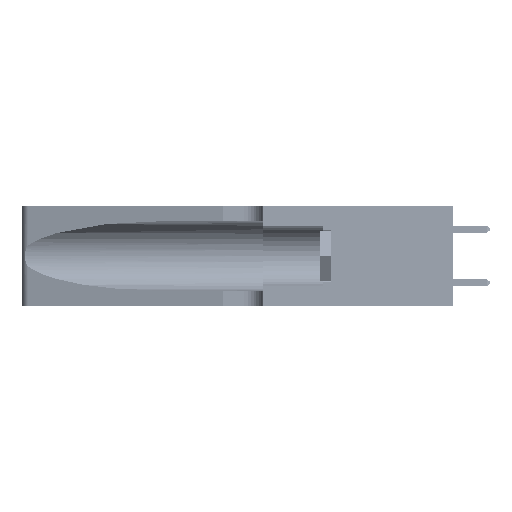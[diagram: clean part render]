
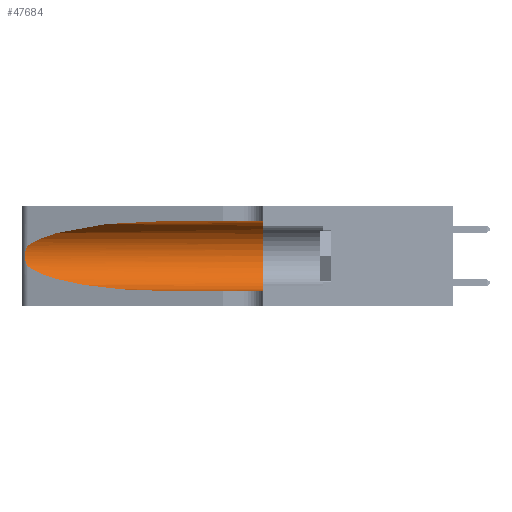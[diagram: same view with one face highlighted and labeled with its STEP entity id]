
A CAD part, left-side view. The second image highlights one B-rep face of the part: STEP entity #47684.
In plain terms, the highlighted cylindrical face has radius 3.308 mm (diameter 6.617 mm), a partial arc.
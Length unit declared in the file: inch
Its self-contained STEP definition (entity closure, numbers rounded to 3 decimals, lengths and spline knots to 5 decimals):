
#236 = CARTESIAN_POINT ( 'NONE',  ( 0.26017, 1.23833, 0.17102 ) ) ;
#421 = CARTESIAN_POINT ( 'NONE',  ( 0.1305, 0.72297, 0.31525 ) ) ;
#479 = DIRECTION ( 'NONE',  ( 0., -1., 0. ) ) ;
#1711 = EDGE_LOOP ( 'NONE', ( #21023, #47205, #43191, #45791, #19119, #29089 ) ) ;
#2213 = CARTESIAN_POINT ( 'NONE',  ( 0.18966, 0.96281, 0.31525 ) ) ;
#3216 = AXIS2_PLACEMENT_3D ( 'NONE', #35411, #479, #12188 ) ;
#3513 = CARTESIAN_POINT ( 'NONE',  ( 0.25487, 1.22718, 0.14631 ) ) ;
#4180 = CARTESIAN_POINT ( 'NONE',  ( 0.25789, 1.23486, 0.15765 ) ) ;
#4497 = CYLINDRICAL_SURFACE ( 'NONE', #3216, 0.13025 ) ;
#6100 = CARTESIAN_POINT ( 'NONE',  ( 0.2373, 1.15595, 0.28018 ) ) ;
#7120 = CARTESIAN_POINT ( 'NONE',  ( 0.1305, 0.72297, 0.05475 ) ) ;
#7264 = CARTESIAN_POINT ( 'NONE',  ( 0.25487, 1.22718, 0.22369 ) ) ;
#8090 = CARTESIAN_POINT ( 'NONE',  ( 0.25555, 1.22993, 0.14849 ) ) ;
#9442 = VERTEX_POINT ( 'NONE', #41348 ) ;
#12087 = B_SPLINE_CURVE_WITH_KNOTS ( 'NONE', 3,
 ( #46562, #38763, #38922, #15696, #42808, #19620, #46723, #23546, #236, #27420, #4180, #31270, #8090, #35182 ),
 .UNSPECIFIED., .F., .F.,
 ( 4, 2, 2, 2, 2, 2, 4 ),
 ( 0., 0.00027, 0.00053, 0.00107, 0.0016, 0.00187, 0.00214 ),
 .UNSPECIFIED. ) ;
#12188 = DIRECTION ( 'NONE',  ( 0., 0., -1. ) ) ;
#12917 = VERTEX_POINT ( 'NONE', #16589 ) ;
#12994 = VECTOR ( 'NONE', #47787, 39.37008 ) ;
#13195 = VERTEX_POINT ( 'NONE', #7264 ) ;
#15198 = CARTESIAN_POINT ( 'NONE',  ( 0.2373, 1.15595, 0.08982 ) ) ;
#15696 = CARTESIAN_POINT ( 'NONE',  ( 0.25787, 1.23484, 0.2124 ) ) ;
#16575 = VECTOR ( 'NONE', #37188, 39.37008 ) ;
#16589 = CARTESIAN_POINT ( 'NONE',  ( 0.25487, 1.22718, 0.14631 ) ) ;
#18305 = CARTESIAN_POINT ( 'NONE',  ( 0.1305, 0.35, 0.31525 ) ) ;
#18373 = CARTESIAN_POINT ( 'NONE',  ( 0.1305, 0.35, 0.185 ) ) ;
#19117 = CARTESIAN_POINT ( 'NONE',  ( 0.1305, 0.72297, 0.05475 ) ) ;
#19119 = ORIENTED_EDGE ( 'NONE', *, *, #24351, .F. ) ;
#19498 = AXIS2_PLACEMENT_3D ( 'NONE', #18373, #45493, #22306 ) ;
#19620 = CARTESIAN_POINT ( 'NONE',  ( 0.26018, 1.23835, 0.19895 ) ) ;
#21023 = ORIENTED_EDGE ( 'NONE', *, *, #45384, .T. ) ;
#22306 = DIRECTION ( 'NONE',  ( 0., 0., 1. ) ) ;
#23546 = CARTESIAN_POINT ( 'NONE',  ( 0.26075, 1.23896, 0.178 ) ) ;
#24351 = EDGE_CURVE ( 'NONE', #26801, #9442, #32994, .T. ) ;
#25138 = VERTEX_POINT ( 'NONE', #7120 ) ;
#25162 = FACE_OUTER_BOUND ( 'NONE', #1711, .T. ) ;
#25484 = CARTESIAN_POINT ( 'NONE',  ( 0.1305, 0.72297, 0.31525 ) ) ;
#25531 = CARTESIAN_POINT ( 'NONE',  ( 0.1305, 1.61858, 0.31525 ) ) ;
#26801 = VERTEX_POINT ( 'NONE', #18305 ) ;
#26916 = LINE ( 'NONE', #25531, #16575 ) ;
#27420 = CARTESIAN_POINT ( 'NONE',  ( 0.25856, 1.23593, 0.16098 ) ) ;
#29089 = ORIENTED_EDGE ( 'NONE', *, *, #48302, .F. ) ;
#30092 =( BOUNDED_CURVE ( )  B_SPLINE_CURVE ( 3, ( #3513, #15198, #42313, #19117 ),
 .UNSPECIFIED., .F., .F. ) 
 B_SPLINE_CURVE_WITH_KNOTS ( ( 4, 4 ),
 ( 3.44316, 4.71239 ),
 .UNSPECIFIED. ) 
 CURVE ( )  GEOMETRIC_REPRESENTATION_ITEM ( )  RATIONAL_B_SPLINE_CURVE ( ( 1., 0.87, 0.87, 1. ) ) 
 REPRESENTATION_ITEM ( '' )  );
#30293 = EDGE_CURVE ( 'NONE', #12917, #25138, #30092, .T. ) ;
#31270 = CARTESIAN_POINT ( 'NONE',  ( 0.25639, 1.23186, 0.15144 ) ) ;
#32994 = CIRCLE ( 'NONE', #19498, 0.13025 ) ;
#33226 = CARTESIAN_POINT ( 'NONE',  ( 0.25487, 1.22718, 0.22369 ) ) ;
#35182 = CARTESIAN_POINT ( 'NONE',  ( 0.25487, 1.22718, 0.14631 ) ) ;
#35384 =( BOUNDED_CURVE ( )  B_SPLINE_CURVE ( 3, ( #25484, #2213, #6100, #33226 ),
 .UNSPECIFIED., .F., .F. ) 
 B_SPLINE_CURVE_WITH_KNOTS ( ( 4, 4 ),
 ( 1.5708, 2.84003 ),
 .UNSPECIFIED. ) 
 CURVE ( )  GEOMETRIC_REPRESENTATION_ITEM ( )  RATIONAL_B_SPLINE_CURVE ( ( 1., 0.87, 0.87, 1. ) ) 
 REPRESENTATION_ITEM ( '' )  );
#35411 = CARTESIAN_POINT ( 'NONE',  ( 0.1305, 1.61858, 0.185 ) ) ;
#37188 = DIRECTION ( 'NONE',  ( 0., -1., 0. ) ) ;
#38360 = EDGE_CURVE ( 'NONE', #13195, #12917, #12087, .T. ) ;
#38763 = CARTESIAN_POINT ( 'NONE',  ( 0.25555, 1.22994, 0.2215 ) ) ;
#38922 = CARTESIAN_POINT ( 'NONE',  ( 0.25639, 1.23184, 0.21858 ) ) ;
#41348 = CARTESIAN_POINT ( 'NONE',  ( 0.1305, 0.35, 0.05475 ) ) ;
#42313 = CARTESIAN_POINT ( 'NONE',  ( 0.18966, 0.96281, 0.05475 ) ) ;
#42808 = CARTESIAN_POINT ( 'NONE',  ( 0.25854, 1.2359, 0.20912 ) ) ;
#43191 = ORIENTED_EDGE ( 'NONE', *, *, #30293, .T. ) ;
#43954 = LINE ( 'NONE', #44049, #12994 ) ;
#44049 = CARTESIAN_POINT ( 'NONE',  ( 0.1305, 1.61858, 0.05475 ) ) ;
#45384 = EDGE_CURVE ( 'NONE', #49933, #13195, #35384, .T. ) ;
#45493 = DIRECTION ( 'NONE',  ( 0., 1., 0. ) ) ;
#45791 = ORIENTED_EDGE ( 'NONE', *, *, #45927, .T. ) ;
#45927 = EDGE_CURVE ( 'NONE', #25138, #9442, #43954, .T. ) ;
#46562 = CARTESIAN_POINT ( 'NONE',  ( 0.25487, 1.22718, 0.22369 ) ) ;
#46723 = CARTESIAN_POINT ( 'NONE',  ( 0.26075, 1.23896, 0.19203 ) ) ;
#47205 = ORIENTED_EDGE ( 'NONE', *, *, #38360, .T. ) ;
#47684 = ADVANCED_FACE ( 'NONE', ( #25162 ), #4497, .F. ) ;
#47787 = DIRECTION ( 'NONE',  ( 0., -1., 0. ) ) ;
#48302 = EDGE_CURVE ( 'NONE', #49933, #26801, #26916, .T. ) ;
#49933 = VERTEX_POINT ( 'NONE', #421 ) ;
